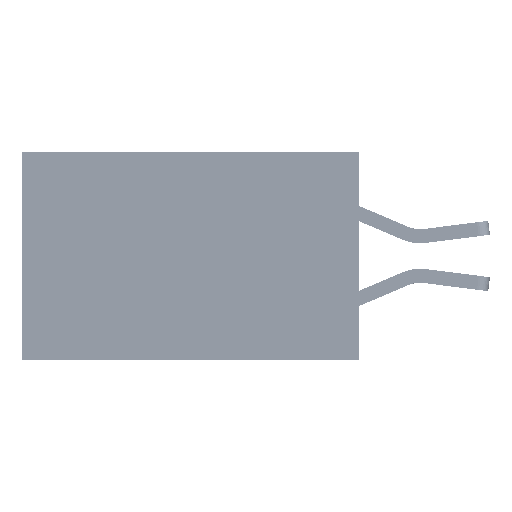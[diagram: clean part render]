
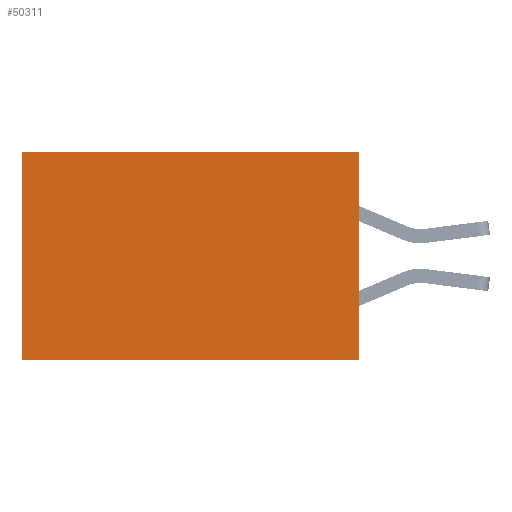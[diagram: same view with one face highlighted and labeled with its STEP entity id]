
A CAD part, left-side view. The second image highlights one B-rep face of the part: STEP entity #50311.
In plain terms, the highlighted planar face has unit normal (-1, 0, 0).
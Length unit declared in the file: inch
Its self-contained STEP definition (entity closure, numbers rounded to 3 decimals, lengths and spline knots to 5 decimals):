
#373 = CARTESIAN_POINT ( 'NONE',  ( 0.2875, 0., -0.37 ) ) ;
#592 = EDGE_CURVE ( 'NONE', #36343, #22287, #33619, .T. ) ;
#649 = CARTESIAN_POINT ( 'NONE',  ( 0.2875, 0.6, 0. ) ) ;
#2061 = EDGE_CURVE ( 'NONE', #22287, #41784, #47488, .T. ) ;
#2983 = CARTESIAN_POINT ( 'NONE',  ( 0.2875, 0.6, -0.37 ) ) ;
#5776 = ORIENTED_EDGE ( 'NONE', *, *, #44173, .F. ) ;
#6163 = VECTOR ( 'NONE', #42755, 39.37008 ) ;
#10667 = ORIENTED_EDGE ( 'NONE', *, *, #2061, .T. ) ;
#11039 = CARTESIAN_POINT ( 'NONE',  ( 0.2875, 0., 0. ) ) ;
#11538 = CARTESIAN_POINT ( 'NONE',  ( 0.2875, 0., 0. ) ) ;
#12298 = DIRECTION ( 'NONE',  ( 0., 0., -1. ) ) ;
#17483 = ORIENTED_EDGE ( 'NONE', *, *, #39956, .F. ) ;
#18680 = EDGE_LOOP ( 'NONE', ( #10667, #17483, #5776, #47618 ) ) ;
#19236 = PLANE ( 'NONE',  #30508 ) ;
#22287 = VERTEX_POINT ( 'NONE', #23817 ) ;
#23292 = LINE ( 'NONE', #373, #6163 ) ;
#23817 = CARTESIAN_POINT ( 'NONE',  ( 0.2875, 0.6, 0. ) ) ;
#24160 = DIRECTION ( 'NONE',  ( 0., 0., -1. ) ) ;
#30508 = AXIS2_PLACEMENT_3D ( 'NONE', #11538, #39321, #24160 ) ;
#30797 = CARTESIAN_POINT ( 'NONE',  ( 0.2875, 0., 0. ) ) ;
#33094 = FACE_OUTER_BOUND ( 'NONE', #18680, .T. ) ;
#33619 = LINE ( 'NONE', #30797, #42756 ) ;
#34607 = DIRECTION ( 'NONE',  ( 0., 0., -1. ) ) ;
#36343 = VERTEX_POINT ( 'NONE', #40986 ) ;
#36623 = VERTEX_POINT ( 'NONE', #38885 ) ;
#38102 = LINE ( 'NONE', #11039, #46649 ) ;
#38433 = DIRECTION ( 'NONE',  ( 0., 1., 0. ) ) ;
#38885 = CARTESIAN_POINT ( 'NONE',  ( 0.2875, 0., -0.37 ) ) ;
#39321 = DIRECTION ( 'NONE',  ( 1., 0., 0. ) ) ;
#39956 = EDGE_CURVE ( 'NONE', #36623, #41784, #23292, .T. ) ;
#40986 = CARTESIAN_POINT ( 'NONE',  ( 0.2875, 0., 0. ) ) ;
#41453 = VECTOR ( 'NONE', #12298, 39.37008 ) ;
#41784 = VERTEX_POINT ( 'NONE', #2983 ) ;
#42755 = DIRECTION ( 'NONE',  ( 0., 1., 0. ) ) ;
#42756 = VECTOR ( 'NONE', #38433, 39.37008 ) ;
#44173 = EDGE_CURVE ( 'NONE', #36343, #36623, #38102, .T. ) ;
#46649 = VECTOR ( 'NONE', #34607, 39.37008 ) ;
#47488 = LINE ( 'NONE', #649, #41453 ) ;
#47618 = ORIENTED_EDGE ( 'NONE', *, *, #592, .T. ) ;
#50311 = ADVANCED_FACE ( 'NONE', ( #33094 ), #19236, .F. ) ;
